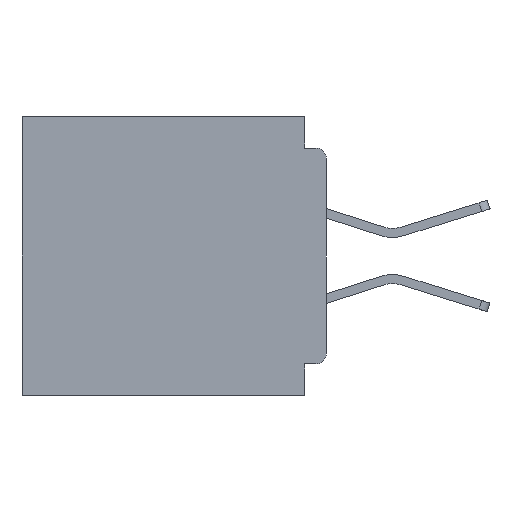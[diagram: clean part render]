
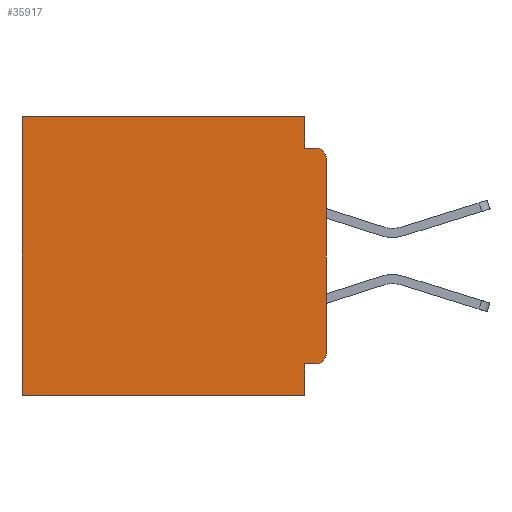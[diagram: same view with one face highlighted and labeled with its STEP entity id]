
A CAD part, left-side view. The second image highlights one B-rep face of the part: STEP entity #35917.
In plain terms, the highlighted planar face has unit normal (-1, 0, 0).
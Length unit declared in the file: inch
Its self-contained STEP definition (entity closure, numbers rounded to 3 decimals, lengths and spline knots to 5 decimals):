
#297 = VERTEX_POINT ( 'NONE', #8649 ) ;
#478 = VERTEX_POINT ( 'NONE', #5200 ) ;
#479 = VECTOR ( 'NONE', #16489, 39.37008 ) ;
#763 = DIRECTION ( 'NONE',  ( 0., 1., 0. ) ) ;
#1225 = FACE_OUTER_BOUND ( 'NONE', #36398, .T. ) ;
#2101 = EDGE_CURVE ( 'NONE', #2994, #478, #5876, .T. ) ;
#2596 = EDGE_CURVE ( 'NONE', #23935, #32475, #28272, .T. ) ;
#2672 = CARTESIAN_POINT ( 'NONE',  ( 0.3, 0.031, 0. ) ) ;
#2994 = VERTEX_POINT ( 'NONE', #14152 ) ;
#3022 = VECTOR ( 'NONE', #38785, 39.37008 ) ;
#3193 = LINE ( 'NONE', #30045, #19889 ) ;
#3503 = VECTOR ( 'NONE', #14983, 39.37008 ) ;
#3533 = EDGE_CURVE ( 'NONE', #23778, #29977, #3193, .T. ) ;
#3982 = VECTOR ( 'NONE', #9052, 39.37008 ) ;
#4083 = LINE ( 'NONE', #38936, #3022 ) ;
#4373 = VECTOR ( 'NONE', #29800, 39.37008 ) ;
#4798 = ORIENTED_EDGE ( 'NONE', *, *, #3533, .T. ) ;
#5117 = CIRCLE ( 'NONE', #25076, 0.015 ) ;
#5152 = VERTEX_POINT ( 'NONE', #28678 ) ;
#5200 = CARTESIAN_POINT ( 'NONE',  ( 0.3, 0., -0.34 ) ) ;
#5291 = EDGE_CURVE ( 'NONE', #32475, #12448, #4083, .T. ) ;
#5876 = LINE ( 'NONE', #32269, #14736 ) ;
#6351 = ORIENTED_EDGE ( 'NONE', *, *, #39268, .T. ) ;
#6354 = DIRECTION ( 'NONE',  ( 1., 0., 0. ) ) ;
#7217 = DIRECTION ( 'NONE',  ( 0., 0., -1. ) ) ;
#8649 = CARTESIAN_POINT ( 'NONE',  ( 0.3, 0.031, -0.045 ) ) ;
#8837 = CARTESIAN_POINT ( 'NONE',  ( 0.3, 0.015, -0.06 ) ) ;
#9009 = ORIENTED_EDGE ( 'NONE', *, *, #2596, .F. ) ;
#9052 = DIRECTION ( 'NONE',  ( 0., 1., 0. ) ) ;
#9621 = CARTESIAN_POINT ( 'NONE',  ( 0.3, 0.031, -0.4 ) ) ;
#12179 = DIRECTION ( 'NONE',  ( 0., 0., -1. ) ) ;
#12448 = VERTEX_POINT ( 'NONE', #12783 ) ;
#12783 = CARTESIAN_POINT ( 'NONE',  ( 0.3, 0.437, -0.4 ) ) ;
#12874 = LINE ( 'NONE', #18972, #3982 ) ;
#13118 = CARTESIAN_POINT ( 'NONE',  ( 0.3, 0.031, 0. ) ) ;
#13137 = ORIENTED_EDGE ( 'NONE', *, *, #2101, .F. ) ;
#13179 = ORIENTED_EDGE ( 'NONE', *, *, #26751, .T. ) ;
#13440 = LINE ( 'NONE', #28270, #3503 ) ;
#13467 = CARTESIAN_POINT ( 'NONE',  ( 0.3, 0.031, -0.355 ) ) ;
#14152 = CARTESIAN_POINT ( 'NONE',  ( 0.3, 0., -0.06 ) ) ;
#14736 = VECTOR ( 'NONE', #28904, 39.37008 ) ;
#14983 = DIRECTION ( 'NONE',  ( 0., 0., -1. ) ) ;
#16489 = DIRECTION ( 'NONE',  ( 0., 0., -1. ) ) ;
#17225 = DIRECTION ( 'NONE',  ( -1., 0., 0. ) ) ;
#18250 = LINE ( 'NONE', #13118, #479 ) ;
#18972 = CARTESIAN_POINT ( 'NONE',  ( 0.3, 0., -0.355 ) ) ;
#19824 = AXIS2_PLACEMENT_3D ( 'NONE', #8837, #32156, #12179 ) ;
#19889 = VECTOR ( 'NONE', #763, 39.37008 ) ;
#20734 = EDGE_CURVE ( 'NONE', #297, #5152, #30990, .T. ) ;
#21499 = ORIENTED_EDGE ( 'NONE', *, *, #38319, .F. ) ;
#23778 = VERTEX_POINT ( 'NONE', #2672 ) ;
#23935 = VERTEX_POINT ( 'NONE', #13467 ) ;
#25076 = AXIS2_PLACEMENT_3D ( 'NONE', #37129, #17225, #40450 ) ;
#26335 = CARTESIAN_POINT ( 'NONE',  ( 0.3, 0., -0.4 ) ) ;
#26446 = CARTESIAN_POINT ( 'NONE',  ( 0.3, 0., -0.045 ) ) ;
#26751 = EDGE_CURVE ( 'NONE', #37307, #478, #5117, .T. ) ;
#27010 = EDGE_CURVE ( 'NONE', #29977, #12448, #13440, .T. ) ;
#27245 = ORIENTED_EDGE ( 'NONE', *, *, #20734, .F. ) ;
#28270 = CARTESIAN_POINT ( 'NONE',  ( 0.3, 0.437, -0.4 ) ) ;
#28272 = LINE ( 'NONE', #37428, #36050 ) ;
#28678 = CARTESIAN_POINT ( 'NONE',  ( 0.3, 0.015, -0.045 ) ) ;
#28904 = DIRECTION ( 'NONE',  ( 0., 0., -1. ) ) ;
#29677 = DIRECTION ( 'NONE',  ( 0., 0., -1. ) ) ;
#29800 = DIRECTION ( 'NONE',  ( 0., -1., 0. ) ) ;
#29977 = VERTEX_POINT ( 'NONE', #37169 ) ;
#30045 = CARTESIAN_POINT ( 'NONE',  ( 0.3, 0., 0. ) ) ;
#30990 = LINE ( 'NONE', #26446, #4373 ) ;
#31424 = ORIENTED_EDGE ( 'NONE', *, *, #27010, .T. ) ;
#32156 = DIRECTION ( 'NONE',  ( -1., 0., 0. ) ) ;
#32269 = CARTESIAN_POINT ( 'NONE',  ( 0.3, 0., -0.4 ) ) ;
#32475 = VERTEX_POINT ( 'NONE', #9621 ) ;
#34301 = EDGE_CURVE ( 'NONE', #37307, #23935, #12874, .T. ) ;
#34517 = ORIENTED_EDGE ( 'NONE', *, *, #5291, .F. ) ;
#35562 = ORIENTED_EDGE ( 'NONE', *, *, #34301, .F. ) ;
#35917 = ADVANCED_FACE ( 'NONE', ( #1225 ), #39544, .F. ) ;
#36050 = VECTOR ( 'NONE', #7217, 39.37008 ) ;
#36398 = EDGE_LOOP ( 'NONE', ( #13137, #6351, #27245, #21499, #4798, #31424, #34517, #9009, #35562, #13179 ) ) ;
#37129 = CARTESIAN_POINT ( 'NONE',  ( 0.3, 0.015, -0.34 ) ) ;
#37169 = CARTESIAN_POINT ( 'NONE',  ( 0.3, 0.437, 0. ) ) ;
#37307 = VERTEX_POINT ( 'NONE', #40591 ) ;
#37428 = CARTESIAN_POINT ( 'NONE',  ( 0.3, 0.031, -0.4 ) ) ;
#37844 = AXIS2_PLACEMENT_3D ( 'NONE', #26335, #6354, #29677 ) ;
#38319 = EDGE_CURVE ( 'NONE', #23778, #297, #18250, .T. ) ;
#38785 = DIRECTION ( 'NONE',  ( 0., 1., 0. ) ) ;
#38936 = CARTESIAN_POINT ( 'NONE',  ( 0.3, 0., -0.4 ) ) ;
#39268 = EDGE_CURVE ( 'NONE', #2994, #5152, #40569, .T. ) ;
#39544 = PLANE ( 'NONE',  #37844 ) ;
#40450 = DIRECTION ( 'NONE',  ( 0., 0., -1. ) ) ;
#40569 = CIRCLE ( 'NONE', #19824, 0.015 ) ;
#40591 = CARTESIAN_POINT ( 'NONE',  ( 0.3, 0.015, -0.355 ) ) ;
